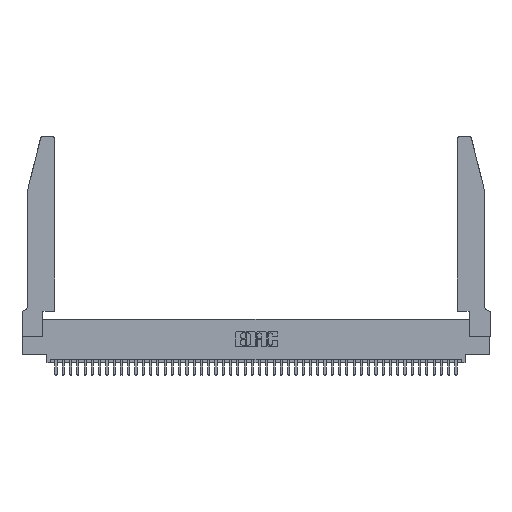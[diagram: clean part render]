
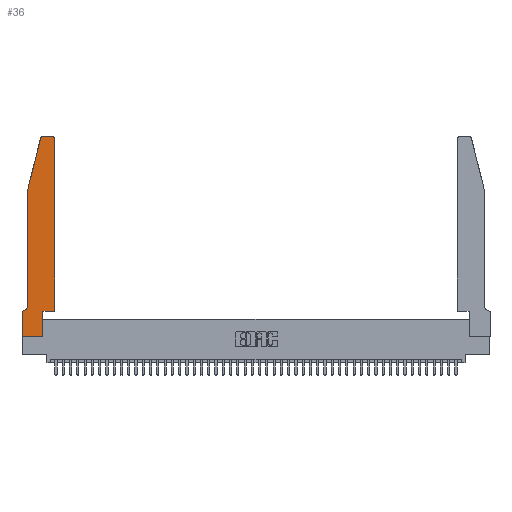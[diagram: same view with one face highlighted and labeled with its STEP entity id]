
A CAD part, top view. The second image highlights one B-rep face of the part: STEP entity #36.
In plain terms, the highlighted planar face has unit normal (0, 0, 1).
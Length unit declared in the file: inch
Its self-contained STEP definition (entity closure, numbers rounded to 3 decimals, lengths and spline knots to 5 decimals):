
#36 = ADVANCED_FACE ( 'NONE', ( #28635 ), #16491, .T. ) ;
#37 = CARTESIAN_POINT ( 'NONE',  ( 0., 0., 0.37 ) ) ;
#220 = VERTEX_POINT ( 'NONE', #44159 ) ;
#1395 = CARTESIAN_POINT ( 'NONE',  ( 0.4205, 2.72, 0.37 ) ) ;
#1485 = EDGE_CURVE ( 'NONE', #26224, #32177, #33078, .T. ) ;
#1562 = DIRECTION ( 'NONE',  ( 1., 0., 0. ) ) ;
#2482 = VECTOR ( 'NONE', #45788, 39.37008 ) ;
#3284 = VECTOR ( 'NONE', #6490, 39.37008 ) ;
#3342 = AXIS2_PLACEMENT_3D ( 'NONE', #23260, #12581, #16450 ) ;
#4169 = VECTOR ( 'NONE', #43513, 39.37008 ) ;
#5180 = EDGE_CURVE ( 'NONE', #12510, #19419, #8720, .T. ) ;
#5526 = CARTESIAN_POINT ( 'NONE',  ( 0., 0.35, 0.37 ) ) ;
#6490 = DIRECTION ( 'NONE',  ( 1., 0., 0. ) ) ;
#6899 = CARTESIAN_POINT ( 'NONE',  ( 0.0755, 2., 0.37 ) ) ;
#8107 = LINE ( 'NONE', #22137, #28036 ) ;
#8720 = LINE ( 'NONE', #46831, #4169 ) ;
#9586 = EDGE_CURVE ( 'NONE', #41978, #26224, #41953, .T. ) ;
#10288 = CARTESIAN_POINT ( 'NONE',  ( 0.2865, 0., 0.37 ) ) ;
#11054 = VERTEX_POINT ( 'NONE', #20283 ) ;
#11608 = ORIENTED_EDGE ( 'NONE', *, *, #12095, .T. ) ;
#12095 = EDGE_CURVE ( 'NONE', #26151, #13629, #41242, .T. ) ;
#12307 = ORIENTED_EDGE ( 'NONE', *, *, #32132, .T. ) ;
#12510 = VERTEX_POINT ( 'NONE', #36611 ) ;
#12581 = DIRECTION ( 'NONE',  ( 0., 0., -1. ) ) ;
#13629 = VERTEX_POINT ( 'NONE', #35366 ) ;
#15326 = AXIS2_PLACEMENT_3D ( 'NONE', #1395, #45312, #1562 ) ;
#15798 = EDGE_LOOP ( 'NONE', ( #45870, #11608, #21408, #17034, #16885, #29613, #19895, #12307, #18994, #22406, #43164, #37132 ) ) ;
#16450 = DIRECTION ( 'NONE',  ( -1., 0., 0. ) ) ;
#16491 = PLANE ( 'NONE',  #28924 ) ;
#16639 = DIRECTION ( 'NONE',  ( 1., 0., 0. ) ) ;
#16885 = ORIENTED_EDGE ( 'NONE', *, *, #44063, .T. ) ;
#16939 = VERTEX_POINT ( 'NONE', #10288 ) ;
#17034 = ORIENTED_EDGE ( 'NONE', *, *, #46299, .T. ) ;
#18355 = VECTOR ( 'NONE', #24020, 39.37008 ) ;
#18396 = VECTOR ( 'NONE', #21255, 39.37008 ) ;
#18994 = ORIENTED_EDGE ( 'NONE', *, *, #38044, .T. ) ;
#19419 = VERTEX_POINT ( 'NONE', #5526 ) ;
#19895 = ORIENTED_EDGE ( 'NONE', *, *, #26980, .T. ) ;
#20283 = CARTESIAN_POINT ( 'NONE',  ( 0.0755, 2., 0.37 ) ) ;
#21169 = LINE ( 'NONE', #38153, #23446 ) ;
#21229 = LINE ( 'NONE', #43355, #18396 ) ;
#21255 = DIRECTION ( 'NONE',  ( -0.239, -0.971, 0. ) ) ;
#21408 = ORIENTED_EDGE ( 'NONE', *, *, #21557, .T. ) ;
#21446 = CARTESIAN_POINT ( 'NONE',  ( 0.284, 2.75, 0.37 ) ) ;
#21557 = EDGE_CURVE ( 'NONE', #13629, #11054, #21229, .T. ) ;
#21611 = CARTESIAN_POINT ( 'NONE',  ( 0.4505, 0.35, 0.37 ) ) ;
#22137 = CARTESIAN_POINT ( 'NONE',  ( 0., 0., 0.37 ) ) ;
#22406 = ORIENTED_EDGE ( 'NONE', *, *, #40426, .T. ) ;
#22839 = CARTESIAN_POINT ( 'NONE',  ( 0.284, 2.72, 0.37 ) ) ;
#22904 = LINE ( 'NONE', #6899, #33690 ) ;
#23081 = CIRCLE ( 'NONE', #3342, 0.07 ) ;
#23170 = DIRECTION ( 'NONE',  ( 1., 0., 0. ) ) ;
#23260 = CARTESIAN_POINT ( 'NONE',  ( 0.0055, 0.42, 0.37 ) ) ;
#23446 = VECTOR ( 'NONE', #31019, 39.37008 ) ;
#23508 = CARTESIAN_POINT ( 'NONE',  ( 0., 0., 0.37 ) ) ;
#24020 = DIRECTION ( 'NONE',  ( 0., 1., 0. ) ) ;
#25917 = DIRECTION ( 'NONE',  ( 1., 0., 0. ) ) ;
#26151 = VERTEX_POINT ( 'NONE', #21446 ) ;
#26224 = VERTEX_POINT ( 'NONE', #26470 ) ;
#26470 = CARTESIAN_POINT ( 'NONE',  ( 0.4505, 2.72, 0.37 ) ) ;
#26499 = DIRECTION ( 'NONE',  ( 0., 0., 1. ) ) ;
#26980 = EDGE_CURVE ( 'NONE', #19419, #37735, #28046, .T. ) ;
#28036 = VECTOR ( 'NONE', #25917, 39.37008 ) ;
#28046 = LINE ( 'NONE', #23508, #2482 ) ;
#28635 = FACE_OUTER_BOUND ( 'NONE', #15798, .T. ) ;
#28924 = AXIS2_PLACEMENT_3D ( 'NONE', #34740, #38407, #16639 ) ;
#29269 = CARTESIAN_POINT ( 'NONE',  ( 0.4505, 0.35, 0.37 ) ) ;
#29613 = ORIENTED_EDGE ( 'NONE', *, *, #5180, .T. ) ;
#31019 = DIRECTION ( 'NONE',  ( -1., 0., 0. ) ) ;
#32132 = EDGE_CURVE ( 'NONE', #37735, #16939, #8107, .T. ) ;
#32177 = VERTEX_POINT ( 'NONE', #33848 ) ;
#33078 = CIRCLE ( 'NONE', #15326, 0.03 ) ;
#33690 = VECTOR ( 'NONE', #42590, 39.37008 ) ;
#33848 = CARTESIAN_POINT ( 'NONE',  ( 0.4205, 2.75, 0.37 ) ) ;
#34498 = DIRECTION ( 'NONE',  ( 0., 1., 0. ) ) ;
#34740 = CARTESIAN_POINT ( 'NONE',  ( 0., 0.35, 0.37 ) ) ;
#35155 = AXIS2_PLACEMENT_3D ( 'NONE', #22839, #26499, #23170 ) ;
#35366 = CARTESIAN_POINT ( 'NONE',  ( 0.25487, 2.72718, 0.37 ) ) ;
#36611 = CARTESIAN_POINT ( 'NONE',  ( 0.0055, 0.35, 0.37 ) ) ;
#36795 = VECTOR ( 'NONE', #34498, 39.37008 ) ;
#37132 = ORIENTED_EDGE ( 'NONE', *, *, #1485, .T. ) ;
#37735 = VERTEX_POINT ( 'NONE', #37 ) ;
#37942 = EDGE_CURVE ( 'NONE', #32177, #26151, #21169, .T. ) ;
#38044 = EDGE_CURVE ( 'NONE', #16939, #220, #40500, .T. ) ;
#38153 = CARTESIAN_POINT ( 'NONE',  ( 0.2605, 2.75, 0.37 ) ) ;
#38407 = DIRECTION ( 'NONE',  ( 0., 0., 1. ) ) ;
#40426 = EDGE_CURVE ( 'NONE', #220, #41978, #45411, .T. ) ;
#40500 = LINE ( 'NONE', #42327, #18355 ) ;
#41122 = VERTEX_POINT ( 'NONE', #46828 ) ;
#41242 = CIRCLE ( 'NONE', #35155, 0.03 ) ;
#41953 = LINE ( 'NONE', #42000, #36795 ) ;
#41978 = VERTEX_POINT ( 'NONE', #29269 ) ;
#42000 = CARTESIAN_POINT ( 'NONE',  ( 0.4505, 0.35, 0.37 ) ) ;
#42327 = CARTESIAN_POINT ( 'NONE',  ( 0.2865, 0.35, 0.37 ) ) ;
#42590 = DIRECTION ( 'NONE',  ( 0., -1., 0. ) ) ;
#43164 = ORIENTED_EDGE ( 'NONE', *, *, #9586, .T. ) ;
#43355 = CARTESIAN_POINT ( 'NONE',  ( 0.0755, 2., 0.37 ) ) ;
#43513 = DIRECTION ( 'NONE',  ( -1., 0., 0. ) ) ;
#44063 = EDGE_CURVE ( 'NONE', #41122, #12510, #23081, .T. ) ;
#44159 = CARTESIAN_POINT ( 'NONE',  ( 0.2865, 0.35, 0.37 ) ) ;
#45312 = DIRECTION ( 'NONE',  ( 0., 0., 1. ) ) ;
#45411 = LINE ( 'NONE', #21611, #3284 ) ;
#45788 = DIRECTION ( 'NONE',  ( 0., -1., 0. ) ) ;
#45870 = ORIENTED_EDGE ( 'NONE', *, *, #37942, .T. ) ;
#46299 = EDGE_CURVE ( 'NONE', #11054, #41122, #22904, .T. ) ;
#46828 = CARTESIAN_POINT ( 'NONE',  ( 0.0755, 0.42, 0.37 ) ) ;
#46831 = CARTESIAN_POINT ( 'NONE',  ( 0.0755, 0.35, 0.37 ) ) ;
